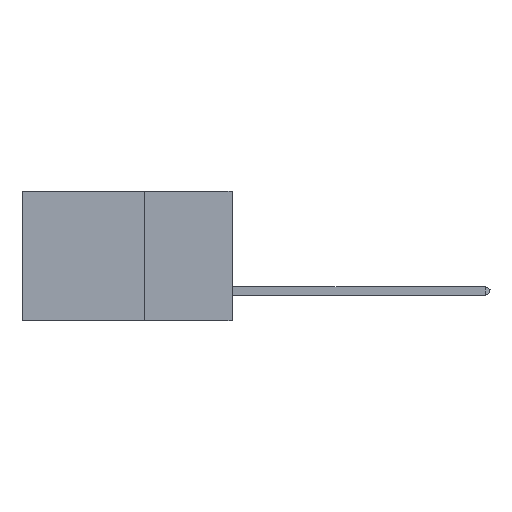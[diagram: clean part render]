
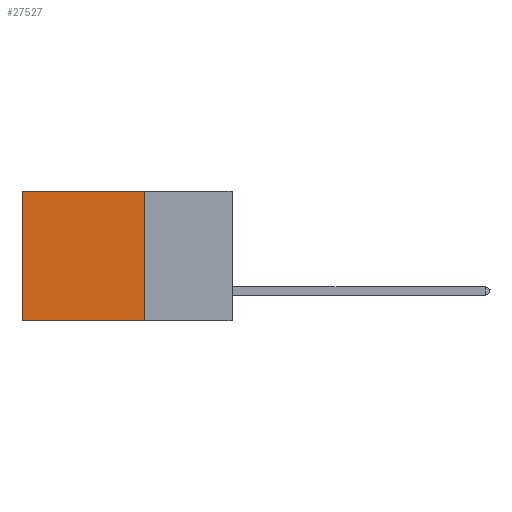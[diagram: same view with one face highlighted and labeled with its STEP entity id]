
A CAD part, left-side view. The second image highlights one B-rep face of the part: STEP entity #27527.
In plain terms, the highlighted planar face has unit normal (-1, 0, 0).
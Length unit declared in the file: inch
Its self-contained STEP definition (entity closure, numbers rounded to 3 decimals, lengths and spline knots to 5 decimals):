
#110 = CARTESIAN_POINT ( 'NONE',  ( 0.2875, 0.6, 0. ) ) ;
#3189 = VECTOR ( 'NONE', #5828, 39.37008 ) ;
#4773 = DIRECTION ( 'NONE',  ( 0., 1., 0. ) ) ;
#4836 = LINE ( 'NONE', #16677, #13320 ) ;
#5472 = VERTEX_POINT ( 'NONE', #31074 ) ;
#5599 = CARTESIAN_POINT ( 'NONE',  ( 0.2875, 0.25, 0. ) ) ;
#5828 = DIRECTION ( 'NONE',  ( 0., 0., -1. ) ) ;
#6779 = DIRECTION ( 'NONE',  ( 0., 0., -1. ) ) ;
#7205 = EDGE_CURVE ( 'NONE', #5472, #31190, #27918, .T. ) ;
#8063 = DIRECTION ( 'NONE',  ( 0., 0., -1. ) ) ;
#8213 = ORIENTED_EDGE ( 'NONE', *, *, #9155, .T. ) ;
#9155 = EDGE_CURVE ( 'NONE', #9511, #5472, #12713, .T. ) ;
#9511 = VERTEX_POINT ( 'NONE', #5599 ) ;
#9704 = EDGE_LOOP ( 'NONE', ( #18004, #31876, #19598, #8213 ) ) ;
#9814 = CARTESIAN_POINT ( 'NONE',  ( 0.2875, 0.6, -0.37 ) ) ;
#12713 = LINE ( 'NONE', #31680, #30088 ) ;
#12947 = DIRECTION ( 'NONE',  ( 1., 0., 0. ) ) ;
#13320 = VECTOR ( 'NONE', #6779, 39.37008 ) ;
#14146 = CARTESIAN_POINT ( 'NONE',  ( 0.2875, 0.25, -0.37 ) ) ;
#16677 = CARTESIAN_POINT ( 'NONE',  ( 0.2875, 0.25, 0. ) ) ;
#16849 = DIRECTION ( 'NONE',  ( 0., 1., 0. ) ) ;
#17583 = AXIS2_PLACEMENT_3D ( 'NONE', #17654, #12947, #8063 ) ;
#17654 = CARTESIAN_POINT ( 'NONE',  ( 0.2875, 0.25, 0. ) ) ;
#18004 = ORIENTED_EDGE ( 'NONE', *, *, #7205, .T. ) ;
#18778 = LINE ( 'NONE', #29485, #22276 ) ;
#19598 = ORIENTED_EDGE ( 'NONE', *, *, #25510, .F. ) ;
#20898 = EDGE_CURVE ( 'NONE', #22866, #31190, #18778, .T. ) ;
#22276 = VECTOR ( 'NONE', #4773, 39.37008 ) ;
#22866 = VERTEX_POINT ( 'NONE', #14146 ) ;
#24908 = PLANE ( 'NONE',  #17583 ) ;
#25510 = EDGE_CURVE ( 'NONE', #9511, #22866, #4836, .T. ) ;
#27527 = ADVANCED_FACE ( 'NONE', ( #29364 ), #24908, .F. ) ;
#27918 = LINE ( 'NONE', #110, #3189 ) ;
#29364 = FACE_OUTER_BOUND ( 'NONE', #9704, .T. ) ;
#29485 = CARTESIAN_POINT ( 'NONE',  ( 0.2875, 0.25, -0.37 ) ) ;
#30088 = VECTOR ( 'NONE', #16849, 39.37008 ) ;
#31074 = CARTESIAN_POINT ( 'NONE',  ( 0.2875, 0.6, 0. ) ) ;
#31190 = VERTEX_POINT ( 'NONE', #9814 ) ;
#31680 = CARTESIAN_POINT ( 'NONE',  ( 0.2875, 0.25, 0. ) ) ;
#31876 = ORIENTED_EDGE ( 'NONE', *, *, #20898, .F. ) ;
